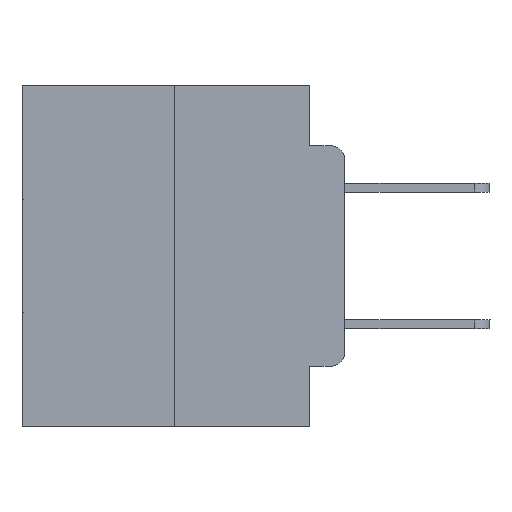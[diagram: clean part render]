
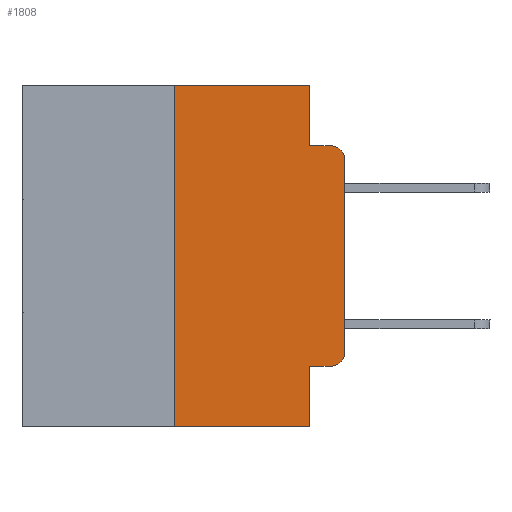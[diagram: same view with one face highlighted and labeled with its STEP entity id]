
A CAD part, left-side view. The second image highlights one B-rep face of the part: STEP entity #1808.
In plain terms, the highlighted planar face has unit normal (-1, 0, 0).
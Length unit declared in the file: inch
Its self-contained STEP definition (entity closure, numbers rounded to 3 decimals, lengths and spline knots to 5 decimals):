
#44 = AXIS2_PLACEMENT_3D ( 'NONE', #13131, #21678, #2406 ) ;
#132 = CARTESIAN_POINT ( 'NONE',  ( 0., 0., 0. ) ) ;
#297 = VERTEX_POINT ( 'NONE', #1713 ) ;
#322 = FACE_OUTER_BOUND ( 'NONE', #8899, .T. ) ;
#335 = LINE ( 'NONE', #2706, #9542 ) ;
#875 = LINE ( 'NONE', #5392, #15487 ) ;
#1572 = VERTEX_POINT ( 'NONE', #8214 ) ;
#1713 = CARTESIAN_POINT ( 'NONE',  ( 0., 0.051, -0.4115 ) ) ;
#1808 = ADVANCED_FACE ( 'NONE', ( #322 ), #8635, .F. ) ;
#1841 = CARTESIAN_POINT ( 'NONE',  ( 0., 0.051, 0. ) ) ;
#1950 = DIRECTION ( 'NONE',  ( 0., 0., 1. ) ) ;
#2064 = CARTESIAN_POINT ( 'NONE',  ( 0., 0.473, 0. ) ) ;
#2217 = ORIENTED_EDGE ( 'NONE', *, *, #9250, .T. ) ;
#2406 = DIRECTION ( 'NONE',  ( 0., 0., -1. ) ) ;
#2412 = ORIENTED_EDGE ( 'NONE', *, *, #7575, .F. ) ;
#2706 = CARTESIAN_POINT ( 'NONE',  ( 0., 0.25, 0. ) ) ;
#3857 = VERTEX_POINT ( 'NONE', #20041 ) ;
#4894 = CIRCLE ( 'NONE', #13848, 0.02 ) ;
#4914 = EDGE_CURVE ( 'NONE', #17662, #1572, #16152, .T. ) ;
#5392 = CARTESIAN_POINT ( 'NONE',  ( 0., 0.051, -0.4115 ) ) ;
#5424 = EDGE_CURVE ( 'NONE', #13185, #21793, #9249, .T. ) ;
#5680 = ORIENTED_EDGE ( 'NONE', *, *, #4914, .F. ) ;
#6215 = LINE ( 'NONE', #21252, #16670 ) ;
#6416 = CARTESIAN_POINT ( 'NONE',  ( 0., 0.02, -0.1085 ) ) ;
#6617 = DIRECTION ( 'NONE',  ( 0., -1., 0. ) ) ;
#7034 = VECTOR ( 'NONE', #10442, 39.37008 ) ;
#7575 = EDGE_CURVE ( 'NONE', #1572, #11403, #13893, .T. ) ;
#7618 = ORIENTED_EDGE ( 'NONE', *, *, #13016, .F. ) ;
#7651 = VERTEX_POINT ( 'NONE', #24306 ) ;
#8184 = ORIENTED_EDGE ( 'NONE', *, *, #20852, .F. ) ;
#8214 = CARTESIAN_POINT ( 'NONE',  ( 0., 0.051, -0.0885 ) ) ;
#8454 = LINE ( 'NONE', #132, #20573 ) ;
#8635 = PLANE ( 'NONE',  #44 ) ;
#8802 = CARTESIAN_POINT ( 'NONE',  ( 0., 0.051, -0.5 ) ) ;
#8899 = EDGE_LOOP ( 'NONE', ( #2217, #23703, #2412, #5680, #21393, #8184, #13339, #7618, #17364, #10971 ) ) ;
#9249 = CIRCLE ( 'NONE', #22704, 0.02 ) ;
#9250 = EDGE_CURVE ( 'NONE', #21793, #7651, #8454, .T. ) ;
#9542 = VECTOR ( 'NONE', #15380, 39.37008 ) ;
#10442 = DIRECTION ( 'NONE',  ( 0., 0., -1. ) ) ;
#10971 = ORIENTED_EDGE ( 'NONE', *, *, #5424, .T. ) ;
#11354 = EDGE_CURVE ( 'NONE', #297, #13185, #875, .T. ) ;
#11403 = VERTEX_POINT ( 'NONE', #13951 ) ;
#11639 = CARTESIAN_POINT ( 'NONE',  ( 0., 0.051, 0. ) ) ;
#12177 = DIRECTION ( 'NONE',  ( -1., 0., 0. ) ) ;
#12640 = CARTESIAN_POINT ( 'NONE',  ( 0., 0.25, -0.5 ) ) ;
#13016 = EDGE_CURVE ( 'NONE', #297, #25366, #21126, .T. ) ;
#13131 = CARTESIAN_POINT ( 'NONE',  ( 0., 0.473, 0. ) ) ;
#13185 = VERTEX_POINT ( 'NONE', #26732 ) ;
#13339 = ORIENTED_EDGE ( 'NONE', *, *, #19440, .T. ) ;
#13783 = VERTEX_POINT ( 'NONE', #12640 ) ;
#13848 = AXIS2_PLACEMENT_3D ( 'NONE', #6416, #21042, #23408 ) ;
#13893 = LINE ( 'NONE', #19939, #21941 ) ;
#13951 = CARTESIAN_POINT ( 'NONE',  ( 0., 0.02, -0.0885 ) ) ;
#15380 = DIRECTION ( 'NONE',  ( 0., 0., 1. ) ) ;
#15440 = DIRECTION ( 'NONE',  ( 0., -1., 0. ) ) ;
#15487 = VECTOR ( 'NONE', #24774, 39.37008 ) ;
#16015 = DIRECTION ( 'NONE',  ( 0., -1., 0. ) ) ;
#16152 = LINE ( 'NONE', #11639, #25132 ) ;
#16405 = CARTESIAN_POINT ( 'NONE',  ( 0., 0.02, -0.3915 ) ) ;
#16670 = VECTOR ( 'NONE', #6617, 39.37008 ) ;
#16756 = EDGE_CURVE ( 'NONE', #7651, #11403, #4894, .T. ) ;
#16861 = VECTOR ( 'NONE', #15440, 39.37008 ) ;
#17364 = ORIENTED_EDGE ( 'NONE', *, *, #11354, .T. ) ;
#17662 = VERTEX_POINT ( 'NONE', #26282 ) ;
#18508 = DIRECTION ( 'NONE',  ( 0., 0., -1. ) ) ;
#19199 = CARTESIAN_POINT ( 'NONE',  ( 0., 0., -0.3915 ) ) ;
#19440 = EDGE_CURVE ( 'NONE', #13783, #25366, #6215, .T. ) ;
#19939 = CARTESIAN_POINT ( 'NONE',  ( 0., 0.051, -0.0885 ) ) ;
#20041 = CARTESIAN_POINT ( 'NONE',  ( 0., 0.25, 0. ) ) ;
#20573 = VECTOR ( 'NONE', #1950, 39.37008 ) ;
#20852 = EDGE_CURVE ( 'NONE', #13783, #3857, #335, .T. ) ;
#21042 = DIRECTION ( 'NONE',  ( -1., 0., 0. ) ) ;
#21126 = LINE ( 'NONE', #1841, #7034 ) ;
#21252 = CARTESIAN_POINT ( 'NONE',  ( 0., 0.473, -0.5 ) ) ;
#21393 = ORIENTED_EDGE ( 'NONE', *, *, #27505, .F. ) ;
#21486 = LINE ( 'NONE', #2064, #16861 ) ;
#21678 = DIRECTION ( 'NONE',  ( 1., 0., 0. ) ) ;
#21793 = VERTEX_POINT ( 'NONE', #19199 ) ;
#21941 = VECTOR ( 'NONE', #16015, 39.37008 ) ;
#22704 = AXIS2_PLACEMENT_3D ( 'NONE', #16405, #12177, #18508 ) ;
#23408 = DIRECTION ( 'NONE',  ( 0., 0., -1. ) ) ;
#23703 = ORIENTED_EDGE ( 'NONE', *, *, #16756, .T. ) ;
#24306 = CARTESIAN_POINT ( 'NONE',  ( 0., 0., -0.1085 ) ) ;
#24713 = DIRECTION ( 'NONE',  ( 0., 0., -1. ) ) ;
#24774 = DIRECTION ( 'NONE',  ( 0., -1., 0. ) ) ;
#25132 = VECTOR ( 'NONE', #24713, 39.37008 ) ;
#25366 = VERTEX_POINT ( 'NONE', #8802 ) ;
#26282 = CARTESIAN_POINT ( 'NONE',  ( 0., 0.051, 0. ) ) ;
#26732 = CARTESIAN_POINT ( 'NONE',  ( 0., 0.02, -0.4115 ) ) ;
#27505 = EDGE_CURVE ( 'NONE', #3857, #17662, #21486, .T. ) ;
